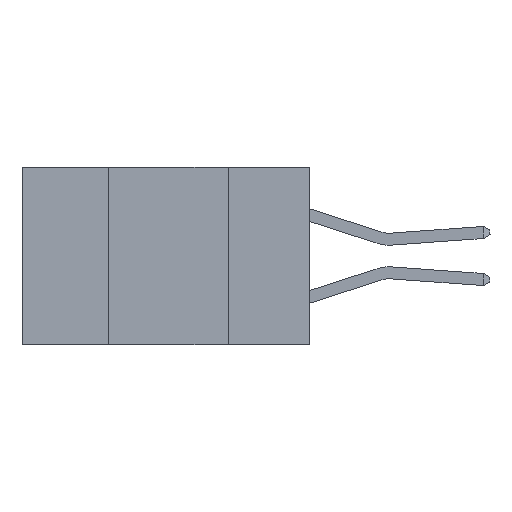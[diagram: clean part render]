
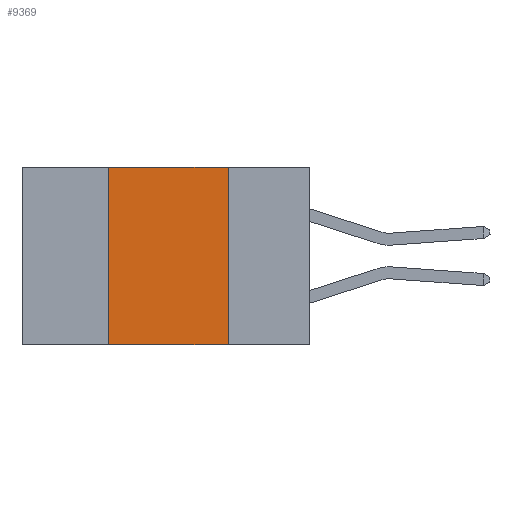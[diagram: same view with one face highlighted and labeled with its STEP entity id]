
A CAD part, left-side view. The second image highlights one B-rep face of the part: STEP entity #9369.
In plain terms, the highlighted planar face has unit normal (-1, 0, 0).
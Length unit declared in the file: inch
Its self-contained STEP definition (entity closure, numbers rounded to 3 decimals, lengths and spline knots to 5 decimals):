
#255 = CARTESIAN_POINT ( 'NONE',  ( 0., 0.17, 0. ) ) ;
#409 = EDGE_CURVE ( 'NONE', #3179, #1270, #14513, .T. ) ;
#1270 = VERTEX_POINT ( 'NONE', #4250 ) ;
#1769 = VECTOR ( 'NONE', #3546, 39.37008 ) ;
#3179 = VERTEX_POINT ( 'NONE', #255 ) ;
#3546 = DIRECTION ( 'NONE',  ( 0., -1., 0. ) ) ;
#3617 = CARTESIAN_POINT ( 'NONE',  ( 0., 0.6, -0.37 ) ) ;
#4250 = CARTESIAN_POINT ( 'NONE',  ( 0., 0.17, -0.37 ) ) ;
#4404 = CARTESIAN_POINT ( 'NONE',  ( 0., 0.42, -0.37 ) ) ;
#4441 = DIRECTION ( 'NONE',  ( 0., 0., 1. ) ) ;
#4941 = VECTOR ( 'NONE', #8228, 39.37008 ) ;
#5546 = ORIENTED_EDGE ( 'NONE', *, *, #9465, .F. ) ;
#6295 = ORIENTED_EDGE ( 'NONE', *, *, #12971, .T. ) ;
#6453 = LINE ( 'NONE', #12898, #10057 ) ;
#7083 = FACE_OUTER_BOUND ( 'NONE', #15328, .T. ) ;
#7304 = DIRECTION ( 'NONE',  ( 0., 0., -1. ) ) ;
#7468 = DIRECTION ( 'NONE',  ( 1., 0., 0. ) ) ;
#7573 = CARTESIAN_POINT ( 'NONE',  ( 0., 0.6, 0. ) ) ;
#7681 = PLANE ( 'NONE',  #12548 ) ;
#8228 = DIRECTION ( 'NONE',  ( 0., 0., -1. ) ) ;
#8971 = CARTESIAN_POINT ( 'NONE',  ( 0., 0.17, -0.37 ) ) ;
#9163 = LINE ( 'NONE', #4404, #11977 ) ;
#9369 = ADVANCED_FACE ( 'NONE', ( #7083 ), #7681, .F. ) ;
#9465 = EDGE_CURVE ( 'NONE', #14402, #13756, #9163, .T. ) ;
#10057 = VECTOR ( 'NONE', #13086, 39.37008 ) ;
#11351 = EDGE_CURVE ( 'NONE', #13756, #3179, #6453, .T. ) ;
#11747 = CARTESIAN_POINT ( 'NONE',  ( 0., 0.42, -0.37 ) ) ;
#11858 = LINE ( 'NONE', #3617, #1769 ) ;
#11977 = VECTOR ( 'NONE', #4441, 39.37008 ) ;
#11980 = ORIENTED_EDGE ( 'NONE', *, *, #409, .F. ) ;
#12144 = ORIENTED_EDGE ( 'NONE', *, *, #11351, .F. ) ;
#12153 = CARTESIAN_POINT ( 'NONE',  ( 0., 0.42, 0. ) ) ;
#12548 = AXIS2_PLACEMENT_3D ( 'NONE', #7573, #7468, #7304 ) ;
#12898 = CARTESIAN_POINT ( 'NONE',  ( 0., 0.6, 0. ) ) ;
#12971 = EDGE_CURVE ( 'NONE', #14402, #1270, #11858, .T. ) ;
#13086 = DIRECTION ( 'NONE',  ( 0., -1., 0. ) ) ;
#13756 = VERTEX_POINT ( 'NONE', #12153 ) ;
#14402 = VERTEX_POINT ( 'NONE', #11747 ) ;
#14513 = LINE ( 'NONE', #8971, #4941 ) ;
#15328 = EDGE_LOOP ( 'NONE', ( #11980, #12144, #5546, #6295 ) ) ;
